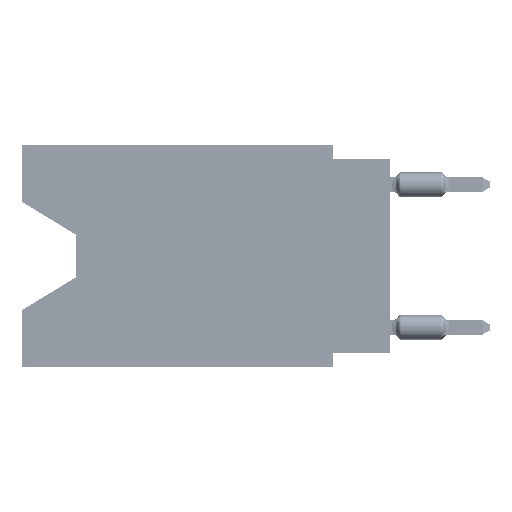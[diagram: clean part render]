
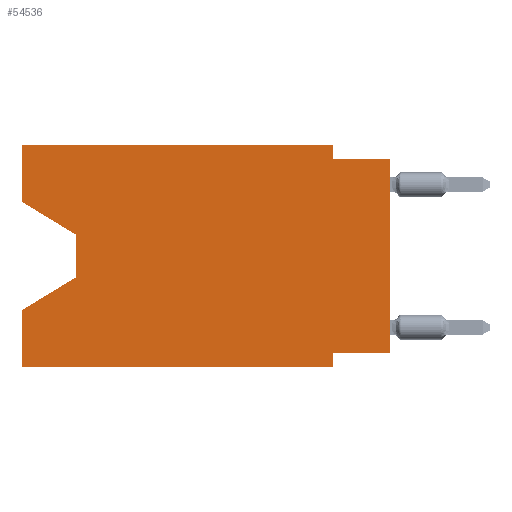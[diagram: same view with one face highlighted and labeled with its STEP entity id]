
A CAD part, left-side view. The second image highlights one B-rep face of the part: STEP entity #54536.
In plain terms, the highlighted planar face has unit normal (-1, 0, 0).
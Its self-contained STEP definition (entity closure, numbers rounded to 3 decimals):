
#962 = EDGE_CURVE ( 'NONE', #10349, #6650, #60880, .T. ) ;
#2031 = VECTOR ( 'NONE', #41261, 1000. ) ;
#2060 = CARTESIAN_POINT ( 'NONE',  ( 0., 2.54, -0.635 ) ) ;
#3469 = DIRECTION ( 'NONE',  ( 0., 0., -1. ) ) ;
#6650 = VERTEX_POINT ( 'NONE', #81433 ) ;
#6719 = CARTESIAN_POINT ( 'NONE',  ( 0., 16.383, -9.906 ) ) ;
#8719 = VERTEX_POINT ( 'NONE', #15517 ) ;
#8745 = EDGE_CURVE ( 'NONE', #42827, #69462, #75806, .T. ) ;
#10349 = VERTEX_POINT ( 'NONE', #40253 ) ;
#10477 = EDGE_LOOP ( 'NONE', ( #18475, #75538, #79591, #36553, #18781, #32774, #25168, #85786, #31700, #25505, #38948, #72049 ) ) ;
#11198 = CARTESIAN_POINT ( 'NONE',  ( 0., 0., -9.271 ) ) ;
#11316 = VECTOR ( 'NONE', #18631, 1000. ) ;
#11635 = DIRECTION ( 'NONE',  ( 0., 1., 0. ) ) ;
#12942 = VECTOR ( 'NONE', #87801, 1000. ) ;
#13870 = LINE ( 'NONE', #75908, #2031 ) ;
#15517 = CARTESIAN_POINT ( 'NONE',  ( 0., 0., -9.271 ) ) ;
#17302 = DIRECTION ( 'NONE',  ( 0., 0., 1. ) ) ;
#17321 = LINE ( 'NONE', #31707, #27232 ) ;
#17334 = VERTEX_POINT ( 'NONE', #38059 ) ;
#17752 = CARTESIAN_POINT ( 'NONE',  ( 0., 16.383, 0. ) ) ;
#18475 = ORIENTED_EDGE ( 'NONE', *, *, #78358, .T. ) ;
#18631 = DIRECTION ( 'NONE',  ( 0., 0.855, -0.519 ) ) ;
#18781 = ORIENTED_EDGE ( 'NONE', *, *, #33890, .T. ) ;
#19949 = CARTESIAN_POINT ( 'NONE',  ( 0., 2.54, -9.906 ) ) ;
#23279 = VECTOR ( 'NONE', #17302, 1000. ) ;
#24074 = LINE ( 'NONE', #39766, #23279 ) ;
#24242 = EDGE_CURVE ( 'NONE', #78740, #56050, #68169, .T. ) ;
#25168 = ORIENTED_EDGE ( 'NONE', *, *, #32005, .F. ) ;
#25505 = ORIENTED_EDGE ( 'NONE', *, *, #24242, .F. ) ;
#27232 = VECTOR ( 'NONE', #44731, 1000. ) ;
#27670 = CARTESIAN_POINT ( 'NONE',  ( 0., 16.383, -7.36 ) ) ;
#27683 = VECTOR ( 'NONE', #69194, 1000. ) ;
#29254 = AXIS2_PLACEMENT_3D ( 'NONE', #57858, #65502, #3469 ) ;
#29727 = VERTEX_POINT ( 'NONE', #27670 ) ;
#31700 = ORIENTED_EDGE ( 'NONE', *, *, #46359, .F. ) ;
#31707 = CARTESIAN_POINT ( 'NONE',  ( 0., 16.383, 0. ) ) ;
#32005 = EDGE_CURVE ( 'NONE', #8719, #10349, #53433, .T. ) ;
#32774 = ORIENTED_EDGE ( 'NONE', *, *, #962, .F. ) ;
#33674 = VECTOR ( 'NONE', #63430, 1000. ) ;
#33812 = LINE ( 'NONE', #82384, #11316 ) ;
#33890 = EDGE_CURVE ( 'NONE', #43615, #6650, #40387, .T. ) ;
#34868 = DIRECTION ( 'NONE',  ( 0., 0., -1. ) ) ;
#36443 = CARTESIAN_POINT ( 'NONE',  ( 0., 16.383, -2.546 ) ) ;
#36553 = ORIENTED_EDGE ( 'NONE', *, *, #71870, .F. ) ;
#38059 = CARTESIAN_POINT ( 'NONE',  ( 0., 0., -0.635 ) ) ;
#38717 = VERTEX_POINT ( 'NONE', #69322 ) ;
#38948 = ORIENTED_EDGE ( 'NONE', *, *, #40986, .F. ) ;
#39588 = VECTOR ( 'NONE', #60990, 1000. ) ;
#39766 = CARTESIAN_POINT ( 'NONE',  ( 0., 0., 0. ) ) ;
#39806 = EDGE_CURVE ( 'NONE', #69462, #29727, #33812, .T. ) ;
#39842 = LINE ( 'NONE', #67730, #39588 ) ;
#40253 = CARTESIAN_POINT ( 'NONE',  ( 0., 2.54, -9.271 ) ) ;
#40387 = LINE ( 'NONE', #6719, #27683 ) ;
#40414 = CARTESIAN_POINT ( 'NONE',  ( 0., 13.97, -4.013 ) ) ;
#40573 = VECTOR ( 'NONE', #11635, 1000. ) ;
#40986 = EDGE_CURVE ( 'NONE', #70208, #78740, #17321, .T. ) ;
#41261 = DIRECTION ( 'NONE',  ( 0., -1., 0. ) ) ;
#42827 = VERTEX_POINT ( 'NONE', #40414 ) ;
#43615 = VERTEX_POINT ( 'NONE', #78057 ) ;
#44340 = PLANE ( 'NONE',  #29254 ) ;
#44731 = DIRECTION ( 'NONE',  ( 0., -1., 0. ) ) ;
#45233 = FACE_OUTER_BOUND ( 'NONE', #10477, .T. ) ;
#46359 = EDGE_CURVE ( 'NONE', #56050, #17334, #13870, .T. ) ;
#47349 = DIRECTION ( 'NONE',  ( 0., 0., -1. ) ) ;
#50082 = CARTESIAN_POINT ( 'NONE',  ( 0., 13.97, -4.013 ) ) ;
#53433 = LINE ( 'NONE', #11198, #40573 ) ;
#54536 = ADVANCED_FACE ( 'NONE', ( #45233 ), #44340, .F. ) ;
#56050 = VERTEX_POINT ( 'NONE', #2060 ) ;
#57858 = CARTESIAN_POINT ( 'NONE',  ( 0., 16.383, 0. ) ) ;
#59928 = LINE ( 'NONE', #80171, #12942 ) ;
#60662 = CARTESIAN_POINT ( 'NONE',  ( 0., 13.97, -5.893 ) ) ;
#60880 = LINE ( 'NONE', #19949, #83751 ) ;
#60990 = DIRECTION ( 'NONE',  ( 0., 0., 1. ) ) ;
#61799 = VECTOR ( 'NONE', #34868, 1000. ) ;
#62752 = DIRECTION ( 'NONE',  ( 0., 0., -1. ) ) ;
#63430 = DIRECTION ( 'NONE',  ( 0., -0.855, -0.519 ) ) ;
#65502 = DIRECTION ( 'NONE',  ( 1., 0., 0. ) ) ;
#66651 = EDGE_CURVE ( 'NONE', #38717, #70208, #39842, .T. ) ;
#67730 = CARTESIAN_POINT ( 'NONE',  ( 0., 16.383, 0. ) ) ;
#68169 = LINE ( 'NONE', #82561, #61799 ) ;
#69194 = DIRECTION ( 'NONE',  ( 0., -1., 0. ) ) ;
#69322 = CARTESIAN_POINT ( 'NONE',  ( 0., 16.383, -2.546 ) ) ;
#69462 = VERTEX_POINT ( 'NONE', #60662 ) ;
#70208 = VERTEX_POINT ( 'NONE', #17752 ) ;
#71870 = EDGE_CURVE ( 'NONE', #43615, #29727, #59928, .T. ) ;
#72049 = ORIENTED_EDGE ( 'NONE', *, *, #66651, .F. ) ;
#74406 = EDGE_CURVE ( 'NONE', #8719, #17334, #24074, .T. ) ;
#75538 = ORIENTED_EDGE ( 'NONE', *, *, #8745, .T. ) ;
#75806 = LINE ( 'NONE', #50082, #87466 ) ;
#75908 = CARTESIAN_POINT ( 'NONE',  ( 0., 0., -0.635 ) ) ;
#77815 = LINE ( 'NONE', #36443, #33674 ) ;
#78057 = CARTESIAN_POINT ( 'NONE',  ( 0., 16.383, -9.906 ) ) ;
#78358 = EDGE_CURVE ( 'NONE', #38717, #42827, #77815, .T. ) ;
#78740 = VERTEX_POINT ( 'NONE', #84038 ) ;
#79591 = ORIENTED_EDGE ( 'NONE', *, *, #39806, .T. ) ;
#80171 = CARTESIAN_POINT ( 'NONE',  ( 0., 16.383, 0. ) ) ;
#81433 = CARTESIAN_POINT ( 'NONE',  ( 0., 2.54, -9.906 ) ) ;
#82384 = CARTESIAN_POINT ( 'NONE',  ( 0., 13.97, -5.893 ) ) ;
#82561 = CARTESIAN_POINT ( 'NONE',  ( 0., 2.54, 0. ) ) ;
#83751 = VECTOR ( 'NONE', #47349, 1000. ) ;
#84038 = CARTESIAN_POINT ( 'NONE',  ( 0., 2.54, 0. ) ) ;
#85786 = ORIENTED_EDGE ( 'NONE', *, *, #74406, .T. ) ;
#87466 = VECTOR ( 'NONE', #62752, 1000. ) ;
#87801 = DIRECTION ( 'NONE',  ( 0., 0., 1. ) ) ;
